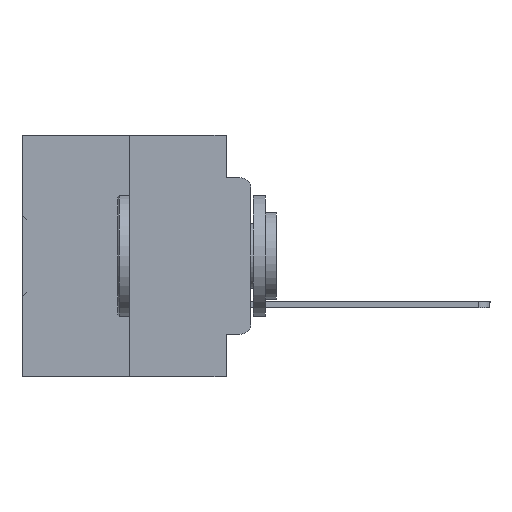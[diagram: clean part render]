
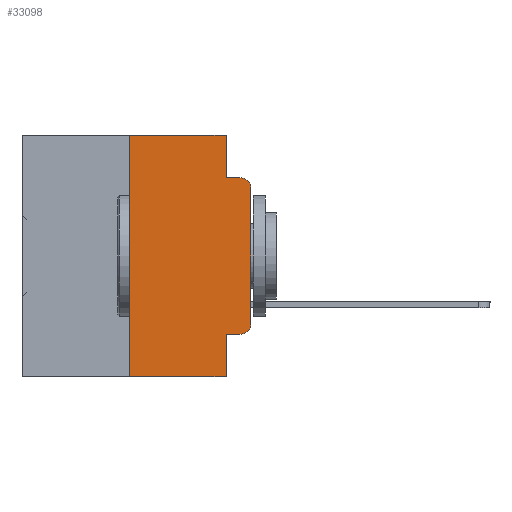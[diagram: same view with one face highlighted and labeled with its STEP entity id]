
A CAD part, left-side view. The second image highlights one B-rep face of the part: STEP entity #33098.
In plain terms, the highlighted planar face has unit normal (-1, 0, 0).
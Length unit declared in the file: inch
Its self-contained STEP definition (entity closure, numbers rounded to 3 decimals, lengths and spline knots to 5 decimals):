
#30 = ORIENTED_EDGE ( 'NONE', *, *, #25101, .T. ) ;
#150 = VECTOR ( 'NONE', #20773, 39.37008 ) ;
#745 = CARTESIAN_POINT ( 'NONE',  ( 0., 0.02, -0.0885 ) ) ;
#799 = CARTESIAN_POINT ( 'NONE',  ( 0., 0.051, 0. ) ) ;
#864 = ORIENTED_EDGE ( 'NONE', *, *, #24795, .F. ) ;
#1094 = LINE ( 'NONE', #35579, #36326 ) ;
#1337 = VERTEX_POINT ( 'NONE', #16320 ) ;
#2001 = DIRECTION ( 'NONE',  ( 1., 0., 0. ) ) ;
#2075 = EDGE_CURVE ( 'NONE', #36222, #13789, #18378, .T. ) ;
#2481 = DIRECTION ( 'NONE',  ( 0., 0., -1. ) ) ;
#2769 = CARTESIAN_POINT ( 'NONE',  ( 0., 0.02, -0.4115 ) ) ;
#3233 = ORIENTED_EDGE ( 'NONE', *, *, #31328, .F. ) ;
#3334 = CARTESIAN_POINT ( 'NONE',  ( 0., 0., -0.3915 ) ) ;
#3437 = CARTESIAN_POINT ( 'NONE',  ( 0., 0.473, -0.5 ) ) ;
#3771 = CARTESIAN_POINT ( 'NONE',  ( 0., 0.051, -0.4115 ) ) ;
#4082 = CARTESIAN_POINT ( 'NONE',  ( 0., 0.25, 0. ) ) ;
#4421 = PLANE ( 'NONE',  #12837 ) ;
#5370 = CARTESIAN_POINT ( 'NONE',  ( 0., 0.051, -0.0885 ) ) ;
#5428 = CARTESIAN_POINT ( 'NONE',  ( 0., 0.051, 0. ) ) ;
#5976 = DIRECTION ( 'NONE',  ( 0., 0., -1. ) ) ;
#6214 = LINE ( 'NONE', #3771, #16918 ) ;
#7374 = ORIENTED_EDGE ( 'NONE', *, *, #19636, .T. ) ;
#8523 = EDGE_CURVE ( 'NONE', #8557, #9549, #8618, .T. ) ;
#8557 = VERTEX_POINT ( 'NONE', #22334 ) ;
#8592 = ORIENTED_EDGE ( 'NONE', *, *, #15281, .T. ) ;
#8618 = LINE ( 'NONE', #5428, #30633 ) ;
#8906 = VERTEX_POINT ( 'NONE', #5370 ) ;
#9235 = LINE ( 'NONE', #31742, #22230 ) ;
#9416 = DIRECTION ( 'NONE',  ( -1., 0., 0. ) ) ;
#9549 = VERTEX_POINT ( 'NONE', #9587 ) ;
#9585 = DIRECTION ( 'NONE',  ( 0., -1., 0. ) ) ;
#9587 = CARTESIAN_POINT ( 'NONE',  ( 0., 0.051, -0.5 ) ) ;
#9618 = DIRECTION ( 'NONE',  ( 0., -1., 0. ) ) ;
#9720 = LINE ( 'NONE', #4082, #150 ) ;
#9961 = VERTEX_POINT ( 'NONE', #35027 ) ;
#12393 = AXIS2_PLACEMENT_3D ( 'NONE', #18240, #9416, #21239 ) ;
#12522 = DIRECTION ( 'NONE',  ( 0., 0., 1. ) ) ;
#12837 = AXIS2_PLACEMENT_3D ( 'NONE', #16046, #2001, #29910 ) ;
#12853 = EDGE_CURVE ( 'NONE', #1337, #35119, #9235, .T. ) ;
#12987 = CARTESIAN_POINT ( 'NONE',  ( 0., 0.051, -0.0885 ) ) ;
#13512 = VERTEX_POINT ( 'NONE', #30358 ) ;
#13789 = VERTEX_POINT ( 'NONE', #3334 ) ;
#13900 = DIRECTION ( 'NONE',  ( -1., 0., 0. ) ) ;
#14324 = VECTOR ( 'NONE', #14870, 39.37008 ) ;
#14870 = DIRECTION ( 'NONE',  ( 0., -1., 0. ) ) ;
#15281 = EDGE_CURVE ( 'NONE', #13789, #13512, #1094, .T. ) ;
#16046 = CARTESIAN_POINT ( 'NONE',  ( 0., 0.473, 0. ) ) ;
#16320 = CARTESIAN_POINT ( 'NONE',  ( 0., 0.25, 0. ) ) ;
#16372 = VERTEX_POINT ( 'NONE', #745 ) ;
#16918 = VECTOR ( 'NONE', #9585, 39.37008 ) ;
#18240 = CARTESIAN_POINT ( 'NONE',  ( 0., 0.02, -0.3915 ) ) ;
#18378 = CIRCLE ( 'NONE', #12393, 0.02 ) ;
#18408 = LINE ( 'NONE', #799, #23909 ) ;
#18890 = EDGE_LOOP ( 'NONE', ( #8592, #7374, #864, #36848, #20560, #3233, #20887, #27403, #30, #25386 ) ) ;
#19407 = EDGE_CURVE ( 'NONE', #35119, #8906, #18408, .T. ) ;
#19636 = EDGE_CURVE ( 'NONE', #13512, #16372, #25148, .T. ) ;
#20560 = ORIENTED_EDGE ( 'NONE', *, *, #12853, .F. ) ;
#20773 = DIRECTION ( 'NONE',  ( 0., 0., 1. ) ) ;
#20887 = ORIENTED_EDGE ( 'NONE', *, *, #26392, .T. ) ;
#21239 = DIRECTION ( 'NONE',  ( 0., 0., -1. ) ) ;
#22230 = VECTOR ( 'NONE', #9618, 39.37008 ) ;
#22334 = CARTESIAN_POINT ( 'NONE',  ( 0., 0.051, -0.4115 ) ) ;
#22785 = LINE ( 'NONE', #3437, #14324 ) ;
#23567 = CARTESIAN_POINT ( 'NONE',  ( 0., 0.051, 0. ) ) ;
#23909 = VECTOR ( 'NONE', #35643, 39.37008 ) ;
#23935 = AXIS2_PLACEMENT_3D ( 'NONE', #28332, #13900, #2481 ) ;
#24071 = DIRECTION ( 'NONE',  ( 0., -1., 0. ) ) ;
#24795 = EDGE_CURVE ( 'NONE', #8906, #16372, #33244, .T. ) ;
#25101 = EDGE_CURVE ( 'NONE', #8557, #36222, #6214, .T. ) ;
#25148 = CIRCLE ( 'NONE', #23935, 0.02 ) ;
#25386 = ORIENTED_EDGE ( 'NONE', *, *, #2075, .T. ) ;
#26392 = EDGE_CURVE ( 'NONE', #9961, #9549, #22785, .T. ) ;
#27403 = ORIENTED_EDGE ( 'NONE', *, *, #8523, .F. ) ;
#28332 = CARTESIAN_POINT ( 'NONE',  ( 0., 0.02, -0.1085 ) ) ;
#29910 = DIRECTION ( 'NONE',  ( 0., 0., -1. ) ) ;
#30358 = CARTESIAN_POINT ( 'NONE',  ( 0., 0., -0.1085 ) ) ;
#30633 = VECTOR ( 'NONE', #5976, 39.37008 ) ;
#31328 = EDGE_CURVE ( 'NONE', #9961, #1337, #9720, .T. ) ;
#31742 = CARTESIAN_POINT ( 'NONE',  ( 0., 0.473, 0. ) ) ;
#31885 = VECTOR ( 'NONE', #24071, 39.37008 ) ;
#33098 = ADVANCED_FACE ( 'NONE', ( #33111 ), #4421, .F. ) ;
#33111 = FACE_OUTER_BOUND ( 'NONE', #18890, .T. ) ;
#33244 = LINE ( 'NONE', #12987, #31885 ) ;
#35027 = CARTESIAN_POINT ( 'NONE',  ( 0., 0.25, -0.5 ) ) ;
#35119 = VERTEX_POINT ( 'NONE', #23567 ) ;
#35579 = CARTESIAN_POINT ( 'NONE',  ( 0., 0., 0. ) ) ;
#35643 = DIRECTION ( 'NONE',  ( 0., 0., -1. ) ) ;
#36222 = VERTEX_POINT ( 'NONE', #2769 ) ;
#36326 = VECTOR ( 'NONE', #12522, 39.37008 ) ;
#36848 = ORIENTED_EDGE ( 'NONE', *, *, #19407, .F. ) ;
